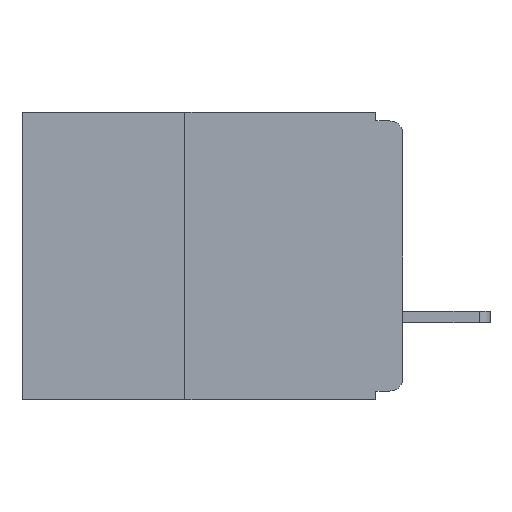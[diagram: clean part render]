
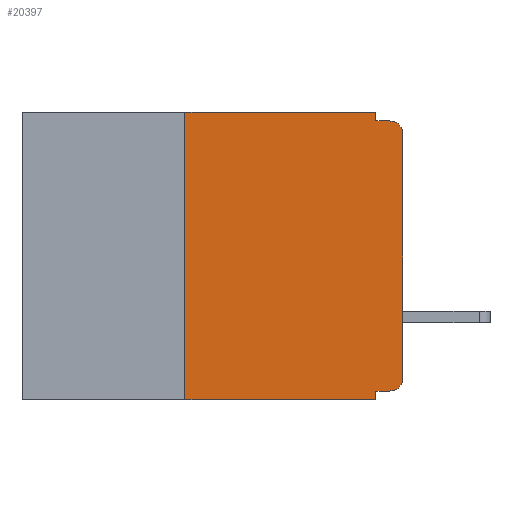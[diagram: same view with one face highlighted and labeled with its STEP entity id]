
A CAD part, left-side view. The second image highlights one B-rep face of the part: STEP entity #20397.
In plain terms, the highlighted planar face has unit normal (-1, 0, 0).
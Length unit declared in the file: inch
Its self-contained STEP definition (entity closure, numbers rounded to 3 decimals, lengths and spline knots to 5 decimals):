
#176 = LINE ( 'NONE', #16341, #25625 ) ;
#755 = VECTOR ( 'NONE', #30580, 39.37008 ) ;
#775 = EDGE_LOOP ( 'NONE', ( #24083, #1334, #16551, #8668, #1551, #3974, #5627, #7484, #10549, #17771 ) ) ;
#1103 = CARTESIAN_POINT ( 'NONE',  ( 0., 0., -0.025 ) ) ;
#1334 = ORIENTED_EDGE ( 'NONE', *, *, #20888, .T. ) ;
#1551 = ORIENTED_EDGE ( 'NONE', *, *, #18117, .F. ) ;
#1770 = CARTESIAN_POINT ( 'NONE',  ( 0., 0.015, -0.01 ) ) ;
#2491 = CARTESIAN_POINT ( 'NONE',  ( 0., 0., -0.305 ) ) ;
#2528 = VECTOR ( 'NONE', #17174, 39.37008 ) ;
#2705 = DIRECTION ( 'NONE',  ( -1., 0., 0. ) ) ;
#3068 = DIRECTION ( 'NONE',  ( -1., 0., 0. ) ) ;
#3138 = VERTEX_POINT ( 'NONE', #1770 ) ;
#3277 = VERTEX_POINT ( 'NONE', #27721 ) ;
#3515 = DIRECTION ( 'NONE',  ( 1., 0., 0. ) ) ;
#3974 = ORIENTED_EDGE ( 'NONE', *, *, #11727, .F. ) ;
#4065 = AXIS2_PLACEMENT_3D ( 'NONE', #17837, #3068, #20318 ) ;
#4542 = LINE ( 'NONE', #29705, #29001 ) ;
#4929 = DIRECTION ( 'NONE',  ( 0., -1., 0. ) ) ;
#5291 = DIRECTION ( 'NONE',  ( 0., 1., 0. ) ) ;
#5627 = ORIENTED_EDGE ( 'NONE', *, *, #23849, .T. ) ;
#5882 = VECTOR ( 'NONE', #28509, 39.37008 ) ;
#6633 = VERTEX_POINT ( 'NONE', #18376 ) ;
#7484 = ORIENTED_EDGE ( 'NONE', *, *, #9794, .F. ) ;
#7527 = VERTEX_POINT ( 'NONE', #22031 ) ;
#8668 = ORIENTED_EDGE ( 'NONE', *, *, #12747, .F. ) ;
#8942 = VECTOR ( 'NONE', #4929, 39.37008 ) ;
#9794 = EDGE_CURVE ( 'NONE', #26848, #3277, #176, .T. ) ;
#10549 = ORIENTED_EDGE ( 'NONE', *, *, #22858, .F. ) ;
#11727 = EDGE_CURVE ( 'NONE', #7527, #6633, #25128, .T. ) ;
#12332 = DIRECTION ( 'NONE',  ( 0., 0., 1. ) ) ;
#12451 = LINE ( 'NONE', #18781, #5882 ) ;
#12747 = EDGE_CURVE ( 'NONE', #30125, #14644, #21263, .T. ) ;
#12837 = EDGE_CURVE ( 'NONE', #30885, #26869, #12451, .T. ) ;
#13393 = CARTESIAN_POINT ( 'NONE',  ( 0., 0.437, 0. ) ) ;
#13603 = AXIS2_PLACEMENT_3D ( 'NONE', #13393, #3515, #20755 ) ;
#14644 = VERTEX_POINT ( 'NONE', #18773 ) ;
#14930 = LINE ( 'NONE', #31599, #2528 ) ;
#15332 = DIRECTION ( 'NONE',  ( 0., -1., 0. ) ) ;
#15867 = CARTESIAN_POINT ( 'NONE',  ( 0., 0.031, -0.32 ) ) ;
#16008 = DIRECTION ( 'NONE',  ( 0., 0., -1. ) ) ;
#16341 = CARTESIAN_POINT ( 'NONE',  ( 0., 0.031, -0.33 ) ) ;
#16551 = ORIENTED_EDGE ( 'NONE', *, *, #20233, .F. ) ;
#16961 = FACE_OUTER_BOUND ( 'NONE', #775, .T. ) ;
#17174 = DIRECTION ( 'NONE',  ( 0., -1., 0. ) ) ;
#17505 = CARTESIAN_POINT ( 'NONE',  ( 0., 0.015, -0.305 ) ) ;
#17771 = ORIENTED_EDGE ( 'NONE', *, *, #19513, .T. ) ;
#17817 = LINE ( 'NONE', #25033, #29934 ) ;
#17837 = CARTESIAN_POINT ( 'NONE',  ( 0., 0.015, -0.025 ) ) ;
#18117 = EDGE_CURVE ( 'NONE', #6633, #30125, #21927, .T. ) ;
#18376 = CARTESIAN_POINT ( 'NONE',  ( 0., 0.25, 0. ) ) ;
#18568 = CARTESIAN_POINT ( 'NONE',  ( 0., 0.031, 0. ) ) ;
#18634 = VECTOR ( 'NONE', #12332, 39.37008 ) ;
#18773 = CARTESIAN_POINT ( 'NONE',  ( 0., 0.031, -0.01 ) ) ;
#18781 = CARTESIAN_POINT ( 'NONE',  ( 0., 0., 0. ) ) ;
#19513 = EDGE_CURVE ( 'NONE', #31211, #30885, #24499, .T. ) ;
#19606 = CARTESIAN_POINT ( 'NONE',  ( 0., 0.25, -0.33 ) ) ;
#19970 = DIRECTION ( 'NONE',  ( 0., 0., -1. ) ) ;
#20233 = EDGE_CURVE ( 'NONE', #14644, #3138, #17817, .T. ) ;
#20318 = DIRECTION ( 'NONE',  ( 0., 0., -1. ) ) ;
#20397 = ADVANCED_FACE ( 'NONE', ( #16961 ), #20656, .F. ) ;
#20656 = PLANE ( 'NONE',  #13603 ) ;
#20755 = DIRECTION ( 'NONE',  ( 0., 0., -1. ) ) ;
#20884 = AXIS2_PLACEMENT_3D ( 'NONE', #17505, #2705, #19970 ) ;
#20888 = EDGE_CURVE ( 'NONE', #26869, #3138, #23117, .T. ) ;
#21263 = LINE ( 'NONE', #18568, #755 ) ;
#21927 = LINE ( 'NONE', #21995, #8942 ) ;
#21995 = CARTESIAN_POINT ( 'NONE',  ( 0., 0.437, 0. ) ) ;
#22031 = CARTESIAN_POINT ( 'NONE',  ( 0., 0.25, -0.33 ) ) ;
#22858 = EDGE_CURVE ( 'NONE', #31211, #26848, #4542, .T. ) ;
#23117 = CIRCLE ( 'NONE', #4065, 0.015 ) ;
#23849 = EDGE_CURVE ( 'NONE', #7527, #3277, #14930, .T. ) ;
#24083 = ORIENTED_EDGE ( 'NONE', *, *, #12837, .T. ) ;
#24499 = CIRCLE ( 'NONE', #20884, 0.015 ) ;
#25033 = CARTESIAN_POINT ( 'NONE',  ( 0., 0., -0.01 ) ) ;
#25128 = LINE ( 'NONE', #19606, #18634 ) ;
#25625 = VECTOR ( 'NONE', #16008, 39.37008 ) ;
#26165 = CARTESIAN_POINT ( 'NONE',  ( 0., 0.031, 0. ) ) ;
#26848 = VERTEX_POINT ( 'NONE', #15867 ) ;
#26869 = VERTEX_POINT ( 'NONE', #1103 ) ;
#27721 = CARTESIAN_POINT ( 'NONE',  ( 0., 0.031, -0.33 ) ) ;
#28176 = CARTESIAN_POINT ( 'NONE',  ( 0., 0.015, -0.32 ) ) ;
#28509 = DIRECTION ( 'NONE',  ( 0., 0., 1. ) ) ;
#29001 = VECTOR ( 'NONE', #5291, 39.37008 ) ;
#29705 = CARTESIAN_POINT ( 'NONE',  ( 0., 0., -0.32 ) ) ;
#29934 = VECTOR ( 'NONE', #15332, 39.37008 ) ;
#30125 = VERTEX_POINT ( 'NONE', #26165 ) ;
#30580 = DIRECTION ( 'NONE',  ( 0., 0., -1. ) ) ;
#30885 = VERTEX_POINT ( 'NONE', #2491 ) ;
#31211 = VERTEX_POINT ( 'NONE', #28176 ) ;
#31599 = CARTESIAN_POINT ( 'NONE',  ( 0., 0.437, -0.33 ) ) ;
